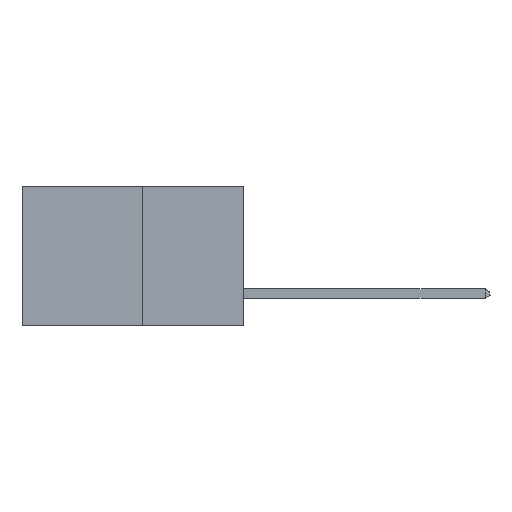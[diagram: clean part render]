
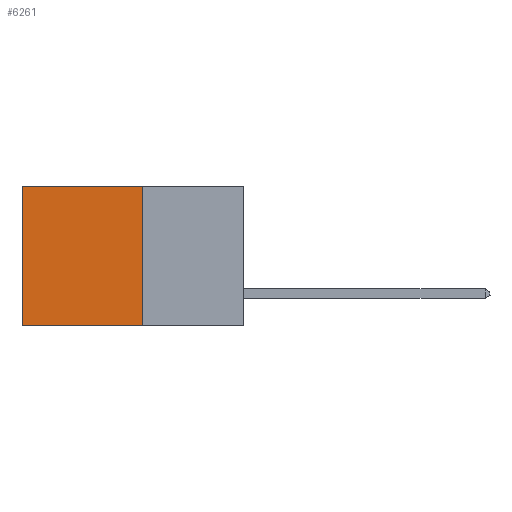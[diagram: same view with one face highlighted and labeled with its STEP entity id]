
A CAD part, left-side view. The second image highlights one B-rep face of the part: STEP entity #6261.
In plain terms, the highlighted planar face has unit normal (-1, 0, 0).
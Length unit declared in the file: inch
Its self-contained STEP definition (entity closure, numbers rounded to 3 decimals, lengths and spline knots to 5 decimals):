
#156 = CARTESIAN_POINT ( 'NONE',  ( 0.277, 0.59, 0. ) ) ;
#586 = AXIS2_PLACEMENT_3D ( 'NONE', #1174, #8329, #3586 ) ;
#604 = CARTESIAN_POINT ( 'NONE',  ( 0.277, 0.27, 0. ) ) ;
#681 = LINE ( 'NONE', #4651, #6522 ) ;
#1156 = VECTOR ( 'NONE', #9938, 39.37008 ) ;
#1174 = CARTESIAN_POINT ( 'NONE',  ( 0.277, 0.27, -0.37 ) ) ;
#1902 = ORIENTED_EDGE ( 'NONE', *, *, #7682, .F. ) ;
#2122 = CARTESIAN_POINT ( 'NONE',  ( 0.277, 0.59, -0.37 ) ) ;
#2326 = CARTESIAN_POINT ( 'NONE',  ( 0.277, 0.27, -0.37 ) ) ;
#3087 = VERTEX_POINT ( 'NONE', #8056 ) ;
#3286 = ORIENTED_EDGE ( 'NONE', *, *, #9733, .T. ) ;
#3445 = CARTESIAN_POINT ( 'NONE',  ( 0.277, 0.27, -0.37 ) ) ;
#3562 = VERTEX_POINT ( 'NONE', #156 ) ;
#3586 = DIRECTION ( 'NONE',  ( 0., 0., -1. ) ) ;
#3707 = DIRECTION ( 'NONE',  ( 0., 0., -1. ) ) ;
#3908 = LINE ( 'NONE', #2326, #7879 ) ;
#4610 = LINE ( 'NONE', #2122, #6715 ) ;
#4651 = CARTESIAN_POINT ( 'NONE',  ( 0.277, 0.27, 0. ) ) ;
#5131 = ORIENTED_EDGE ( 'NONE', *, *, #7137, .T. ) ;
#5295 = CARTESIAN_POINT ( 'NONE',  ( 0.277, 0.27, -0.37 ) ) ;
#6261 = ADVANCED_FACE ( 'NONE', ( #9930 ), #9783, .F. ) ;
#6272 = DIRECTION ( 'NONE',  ( 0., 1., 0. ) ) ;
#6522 = VECTOR ( 'NONE', #8579, 39.37008 ) ;
#6715 = VECTOR ( 'NONE', #3707, 39.37008 ) ;
#6838 = VERTEX_POINT ( 'NONE', #3445 ) ;
#7137 = EDGE_CURVE ( 'NONE', #7607, #3562, #681, .T. ) ;
#7532 = EDGE_CURVE ( 'NONE', #7607, #6838, #9302, .T. ) ;
#7607 = VERTEX_POINT ( 'NONE', #604 ) ;
#7682 = EDGE_CURVE ( 'NONE', #6838, #3087, #3908, .T. ) ;
#7740 = EDGE_LOOP ( 'NONE', ( #3286, #1902, #7882, #5131 ) ) ;
#7879 = VECTOR ( 'NONE', #6272, 39.37008 ) ;
#7882 = ORIENTED_EDGE ( 'NONE', *, *, #7532, .F. ) ;
#8056 = CARTESIAN_POINT ( 'NONE',  ( 0.277, 0.59, -0.37 ) ) ;
#8329 = DIRECTION ( 'NONE',  ( 1., 0., 0. ) ) ;
#8579 = DIRECTION ( 'NONE',  ( 0., 1., 0. ) ) ;
#9302 = LINE ( 'NONE', #5295, #1156 ) ;
#9733 = EDGE_CURVE ( 'NONE', #3562, #3087, #4610, .T. ) ;
#9783 = PLANE ( 'NONE',  #586 ) ;
#9930 = FACE_OUTER_BOUND ( 'NONE', #7740, .T. ) ;
#9938 = DIRECTION ( 'NONE',  ( 0., 0., -1. ) ) ;
